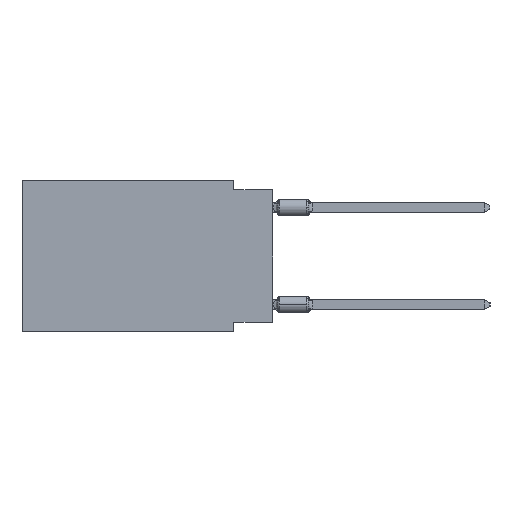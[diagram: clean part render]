
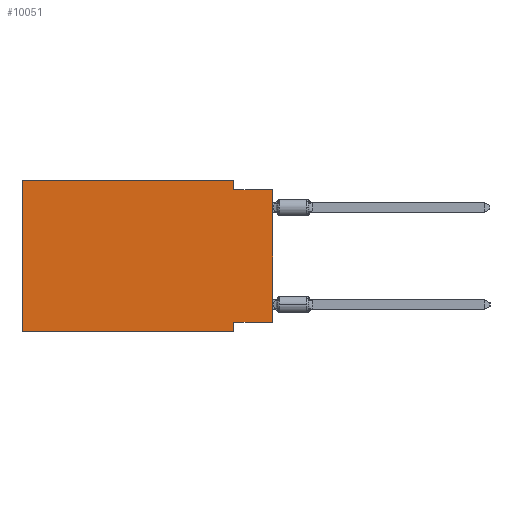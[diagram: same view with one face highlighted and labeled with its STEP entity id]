
A CAD part, left-side view. The second image highlights one B-rep face of the part: STEP entity #10051.
In plain terms, the highlighted planar face has unit normal (-1, 0, 0).
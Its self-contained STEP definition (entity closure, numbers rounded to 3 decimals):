
#161 = VECTOR ( 'NONE', #11364, 1000. ) ;
#1471 = EDGE_CURVE ( 'NONE', #3334, #2895, #21621, .T. ) ;
#2186 = CARTESIAN_POINT ( 'NONE',  ( 0., 16.383, 0. ) ) ;
#2632 = DIRECTION ( 'NONE',  ( 0., 0., 1. ) ) ;
#2895 = VERTEX_POINT ( 'NONE', #60051 ) ;
#3334 = VERTEX_POINT ( 'NONE', #50153 ) ;
#3596 = CARTESIAN_POINT ( 'NONE',  ( 0., 0., -0.635 ) ) ;
#4248 = VECTOR ( 'NONE', #34506, 1000. ) ;
#5075 = DIRECTION ( 'NONE',  ( 0., 0., -1. ) ) ;
#6392 = EDGE_CURVE ( 'NONE', #54428, #31166, #24905, .T. ) ;
#8768 = CARTESIAN_POINT ( 'NONE',  ( 0., 2.54, 0. ) ) ;
#8866 = LINE ( 'NONE', #12855, #14406 ) ;
#9652 = AXIS2_PLACEMENT_3D ( 'NONE', #2186, #16299, #43608 ) ;
#10051 = ADVANCED_FACE ( 'NONE', ( #57405 ), #11399, .F. ) ;
#11044 = EDGE_CURVE ( 'NONE', #32845, #31166, #59359, .T. ) ;
#11364 = DIRECTION ( 'NONE',  ( 0., 0., -1. ) ) ;
#11399 = PLANE ( 'NONE',  #9652 ) ;
#11443 = VECTOR ( 'NONE', #40425, 1000. ) ;
#11936 = ORIENTED_EDGE ( 'NONE', *, *, #12487, .F. ) ;
#12276 = CARTESIAN_POINT ( 'NONE',  ( 0., 16.383, 0. ) ) ;
#12487 = EDGE_CURVE ( 'NONE', #18913, #54428, #50473, .T. ) ;
#12855 = CARTESIAN_POINT ( 'NONE',  ( 0., 0., -9.271 ) ) ;
#14406 = VECTOR ( 'NONE', #27575, 1000. ) ;
#15691 = CARTESIAN_POINT ( 'NONE',  ( 0., 0., -0.635 ) ) ;
#16265 = LINE ( 'NONE', #34361, #161 ) ;
#16299 = DIRECTION ( 'NONE',  ( 1., 0., 0. ) ) ;
#17359 = CARTESIAN_POINT ( 'NONE',  ( 0., 0., 0. ) ) ;
#18863 = DIRECTION ( 'NONE',  ( 0., 0., 1. ) ) ;
#18913 = VERTEX_POINT ( 'NONE', #32500 ) ;
#20857 = ORIENTED_EDGE ( 'NONE', *, *, #1471, .T. ) ;
#21402 = VECTOR ( 'NONE', #18863, 1000. ) ;
#21621 = LINE ( 'NONE', #57815, #4248 ) ;
#21952 = EDGE_CURVE ( 'NONE', #30661, #18913, #39818, .T. ) ;
#24905 = LINE ( 'NONE', #15691, #49655 ) ;
#27575 = DIRECTION ( 'NONE',  ( 0., 1., 0. ) ) ;
#30661 = VERTEX_POINT ( 'NONE', #12276 ) ;
#31166 = VERTEX_POINT ( 'NONE', #3596 ) ;
#31384 = EDGE_LOOP ( 'NONE', ( #35629, #33142, #11936, #32245, #49636, #20857, #54104, #35265 ) ) ;
#31523 = CARTESIAN_POINT ( 'NONE',  ( 0., 16.383, 0. ) ) ;
#32245 = ORIENTED_EDGE ( 'NONE', *, *, #21952, .F. ) ;
#32500 = CARTESIAN_POINT ( 'NONE',  ( 0., 2.54, 0. ) ) ;
#32845 = VERTEX_POINT ( 'NONE', #59647 ) ;
#33142 = ORIENTED_EDGE ( 'NONE', *, *, #6392, .F. ) ;
#34361 = CARTESIAN_POINT ( 'NONE',  ( 0., 2.54, -9.906 ) ) ;
#34506 = DIRECTION ( 'NONE',  ( 0., -1., 0. ) ) ;
#35265 = ORIENTED_EDGE ( 'NONE', *, *, #46604, .F. ) ;
#35629 = ORIENTED_EDGE ( 'NONE', *, *, #11044, .T. ) ;
#38100 = VECTOR ( 'NONE', #5075, 1000. ) ;
#39378 = CARTESIAN_POINT ( 'NONE',  ( 0., 2.54, -9.271 ) ) ;
#39818 = LINE ( 'NONE', #31523, #11443 ) ;
#40425 = DIRECTION ( 'NONE',  ( 0., -1., 0. ) ) ;
#41570 = LINE ( 'NONE', #42174, #21402 ) ;
#41877 = VECTOR ( 'NONE', #2632, 1000. ) ;
#42174 = CARTESIAN_POINT ( 'NONE',  ( 0., 16.383, 0. ) ) ;
#43608 = DIRECTION ( 'NONE',  ( 0., 0., -1. ) ) ;
#46604 = EDGE_CURVE ( 'NONE', #32845, #58438, #8866, .T. ) ;
#49636 = ORIENTED_EDGE ( 'NONE', *, *, #54332, .F. ) ;
#49655 = VECTOR ( 'NONE', #56805, 1000. ) ;
#50153 = CARTESIAN_POINT ( 'NONE',  ( 0., 16.383, -9.906 ) ) ;
#50473 = LINE ( 'NONE', #8768, #38100 ) ;
#53697 = CARTESIAN_POINT ( 'NONE',  ( 0., 2.54, -0.635 ) ) ;
#54104 = ORIENTED_EDGE ( 'NONE', *, *, #59645, .F. ) ;
#54332 = EDGE_CURVE ( 'NONE', #3334, #30661, #41570, .T. ) ;
#54428 = VERTEX_POINT ( 'NONE', #53697 ) ;
#56805 = DIRECTION ( 'NONE',  ( 0., -1., 0. ) ) ;
#57405 = FACE_OUTER_BOUND ( 'NONE', #31384, .T. ) ;
#57815 = CARTESIAN_POINT ( 'NONE',  ( 0., 16.383, -9.906 ) ) ;
#58438 = VERTEX_POINT ( 'NONE', #39378 ) ;
#59359 = LINE ( 'NONE', #17359, #41877 ) ;
#59645 = EDGE_CURVE ( 'NONE', #58438, #2895, #16265, .T. ) ;
#59647 = CARTESIAN_POINT ( 'NONE',  ( 0., 0., -9.271 ) ) ;
#60051 = CARTESIAN_POINT ( 'NONE',  ( 0., 2.54, -9.906 ) ) ;
